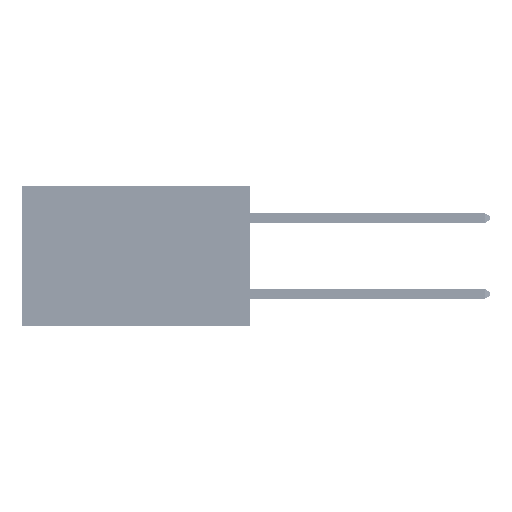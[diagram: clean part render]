
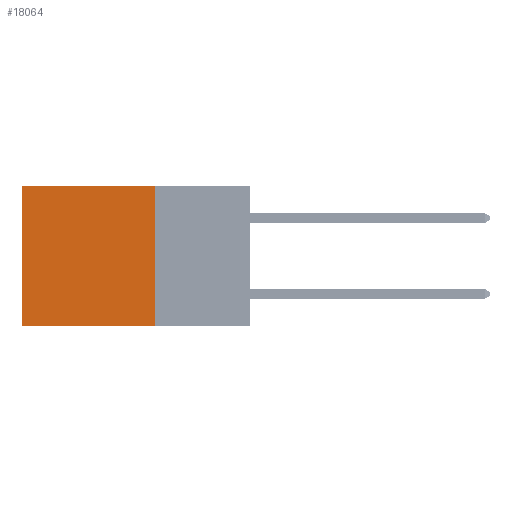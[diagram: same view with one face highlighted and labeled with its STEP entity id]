
A CAD part, left-side view. The second image highlights one B-rep face of the part: STEP entity #18064.
In plain terms, the highlighted planar face has unit normal (-1, 0, 0).
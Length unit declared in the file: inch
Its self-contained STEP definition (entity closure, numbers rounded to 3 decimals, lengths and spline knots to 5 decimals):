
#1125 = CARTESIAN_POINT ( 'NONE',  ( 0.2875, 0.25, 0. ) ) ;
#1362 = VECTOR ( 'NONE', #46600, 39.37008 ) ;
#2761 = VECTOR ( 'NONE', #2905, 39.37008 ) ;
#2905 = DIRECTION ( 'NONE',  ( 0., 0., -1. ) ) ;
#6070 = ORIENTED_EDGE ( 'NONE', *, *, #37611, .T. ) ;
#6631 = EDGE_CURVE ( 'NONE', #36368, #47890, #33296, .T. ) ;
#9836 = CARTESIAN_POINT ( 'NONE',  ( 0.2875, 0.25, -0.37 ) ) ;
#11263 = ORIENTED_EDGE ( 'NONE', *, *, #6631, .F. ) ;
#12395 = DIRECTION ( 'NONE',  ( 0., 1., 0. ) ) ;
#13871 = DIRECTION ( 'NONE',  ( 0., 1., 0. ) ) ;
#15818 = EDGE_LOOP ( 'NONE', ( #31155, #11263, #25096, #6070 ) ) ;
#16631 = DIRECTION ( 'NONE',  ( 1., 0., 0. ) ) ;
#17799 = CARTESIAN_POINT ( 'NONE',  ( 0.2875, 0.6, -0.37 ) ) ;
#18064 = ADVANCED_FACE ( 'NONE', ( #20467 ), #27651, .F. ) ;
#20467 = FACE_OUTER_BOUND ( 'NONE', #15818, .T. ) ;
#24058 = DIRECTION ( 'NONE',  ( 0., 0., -1. ) ) ;
#24428 = CARTESIAN_POINT ( 'NONE',  ( 0.2875, 0.25, 0. ) ) ;
#25096 = ORIENTED_EDGE ( 'NONE', *, *, #47139, .F. ) ;
#26304 = EDGE_CURVE ( 'NONE', #29071, #47890, #43280, .T. ) ;
#27651 = PLANE ( 'NONE',  #44749 ) ;
#29071 = VERTEX_POINT ( 'NONE', #30725 ) ;
#30457 = CARTESIAN_POINT ( 'NONE',  ( 0.2875, 0.25, 0. ) ) ;
#30705 = LINE ( 'NONE', #30457, #2761 ) ;
#30725 = CARTESIAN_POINT ( 'NONE',  ( 0.2875, 0.6, 0. ) ) ;
#31155 = ORIENTED_EDGE ( 'NONE', *, *, #26304, .T. ) ;
#33296 = LINE ( 'NONE', #48799, #39503 ) ;
#36368 = VERTEX_POINT ( 'NONE', #9836 ) ;
#37611 = EDGE_CURVE ( 'NONE', #48991, #29071, #47320, .T. ) ;
#39503 = VECTOR ( 'NONE', #13871, 39.37008 ) ;
#42541 = CARTESIAN_POINT ( 'NONE',  ( 0.2875, 0.6, 0. ) ) ;
#43022 = CARTESIAN_POINT ( 'NONE',  ( 0.2875, 0.25, 0. ) ) ;
#43280 = LINE ( 'NONE', #42541, #1362 ) ;
#43947 = VECTOR ( 'NONE', #12395, 39.37008 ) ;
#44749 = AXIS2_PLACEMENT_3D ( 'NONE', #1125, #16631, #24058 ) ;
#46600 = DIRECTION ( 'NONE',  ( 0., 0., -1. ) ) ;
#47139 = EDGE_CURVE ( 'NONE', #48991, #36368, #30705, .T. ) ;
#47320 = LINE ( 'NONE', #43022, #43947 ) ;
#47890 = VERTEX_POINT ( 'NONE', #17799 ) ;
#48799 = CARTESIAN_POINT ( 'NONE',  ( 0.2875, 0.25, -0.37 ) ) ;
#48991 = VERTEX_POINT ( 'NONE', #24428 ) ;
